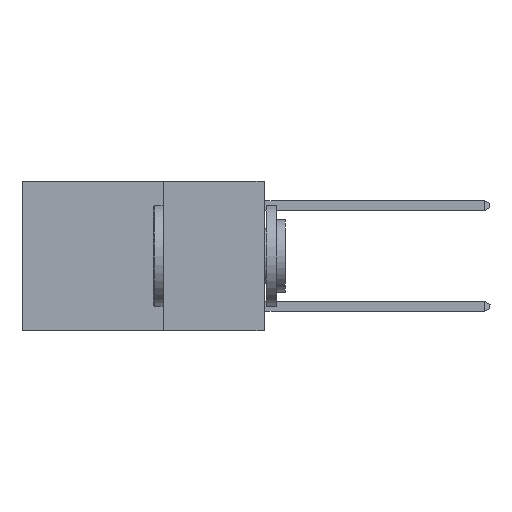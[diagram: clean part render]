
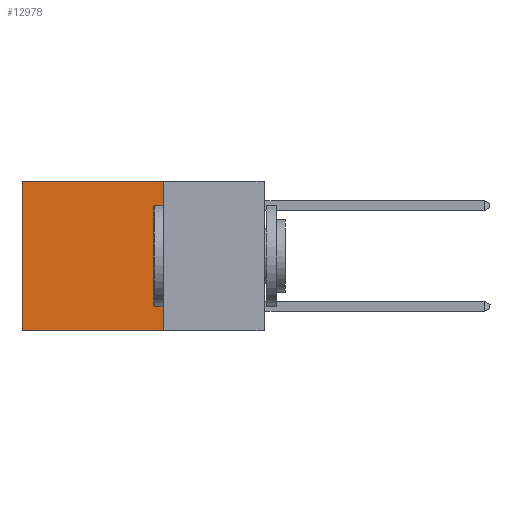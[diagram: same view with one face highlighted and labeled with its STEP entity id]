
A CAD part, left-side view. The second image highlights one B-rep face of the part: STEP entity #12978.
In plain terms, the highlighted planar face has unit normal (-1, 0, 0).
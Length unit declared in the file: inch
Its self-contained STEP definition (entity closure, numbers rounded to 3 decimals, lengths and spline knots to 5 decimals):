
#796 = CARTESIAN_POINT ( 'NONE',  ( 0.2625, 0.25, 0. ) ) ;
#1205 = ORIENTED_EDGE ( 'NONE', *, *, #10169, .F. ) ;
#1776 = FACE_OUTER_BOUND ( 'NONE', #11373, .T. ) ;
#1857 = DIRECTION ( 'NONE',  ( 0., 1., 0. ) ) ;
#3048 = CARTESIAN_POINT ( 'NONE',  ( 0.2625, 0.6, -0.37 ) ) ;
#3402 = ORIENTED_EDGE ( 'NONE', *, *, #9807, .F. ) ;
#5316 = VECTOR ( 'NONE', #26136, 39.37008 ) ;
#5808 = VERTEX_POINT ( 'NONE', #6641 ) ;
#6058 = CARTESIAN_POINT ( 'NONE',  ( 0.2625, 0.25, -0.37 ) ) ;
#6118 = CARTESIAN_POINT ( 'NONE',  ( 0.2625, 0.25, 0. ) ) ;
#6641 = CARTESIAN_POINT ( 'NONE',  ( 0.2625, 0.25, 0. ) ) ;
#7508 = ORIENTED_EDGE ( 'NONE', *, *, #9897, .T. ) ;
#8184 = DIRECTION ( 'NONE',  ( 0., 1., 0. ) ) ;
#8192 = VECTOR ( 'NONE', #1857, 39.37008 ) ;
#8245 = DIRECTION ( 'NONE',  ( 1., 0., 0. ) ) ;
#9807 = EDGE_CURVE ( 'NONE', #5808, #22045, #23976, .T. ) ;
#9897 = EDGE_CURVE ( 'NONE', #26577, #11951, #22677, .T. ) ;
#10169 = EDGE_CURVE ( 'NONE', #22045, #11951, #11867, .T. ) ;
#11238 = CARTESIAN_POINT ( 'NONE',  ( 0.2625, 0.25, -0.37 ) ) ;
#11373 = EDGE_LOOP ( 'NONE', ( #7508, #1205, #3402, #13904 ) ) ;
#11867 = LINE ( 'NONE', #6058, #18114 ) ;
#11951 = VERTEX_POINT ( 'NONE', #3048 ) ;
#12672 = AXIS2_PLACEMENT_3D ( 'NONE', #6118, #8245, #22877 ) ;
#12978 = ADVANCED_FACE ( 'NONE', ( #1776 ), #20781, .F. ) ;
#13904 = ORIENTED_EDGE ( 'NONE', *, *, #16695, .T. ) ;
#14514 = CARTESIAN_POINT ( 'NONE',  ( 0.2625, 0.25, 0. ) ) ;
#15880 = CARTESIAN_POINT ( 'NONE',  ( 0.2625, 0.6, 0. ) ) ;
#16695 = EDGE_CURVE ( 'NONE', #5808, #26577, #26120, .T. ) ;
#18114 = VECTOR ( 'NONE', #8184, 39.37008 ) ;
#18224 = CARTESIAN_POINT ( 'NONE',  ( 0.2625, 0.6, 0. ) ) ;
#18475 = VECTOR ( 'NONE', #19782, 39.37008 ) ;
#19782 = DIRECTION ( 'NONE',  ( 0., 0., -1. ) ) ;
#20781 = PLANE ( 'NONE',  #12672 ) ;
#22045 = VERTEX_POINT ( 'NONE', #11238 ) ;
#22677 = LINE ( 'NONE', #15880, #5316 ) ;
#22877 = DIRECTION ( 'NONE',  ( 0., 0., -1. ) ) ;
#23976 = LINE ( 'NONE', #796, #18475 ) ;
#26120 = LINE ( 'NONE', #14514, #8192 ) ;
#26136 = DIRECTION ( 'NONE',  ( 0., 0., -1. ) ) ;
#26577 = VERTEX_POINT ( 'NONE', #18224 ) ;
